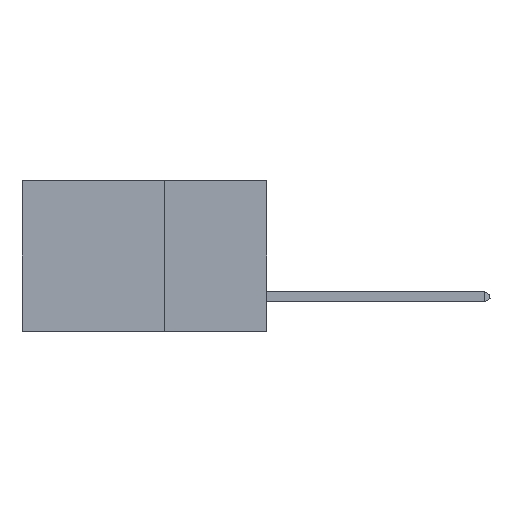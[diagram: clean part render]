
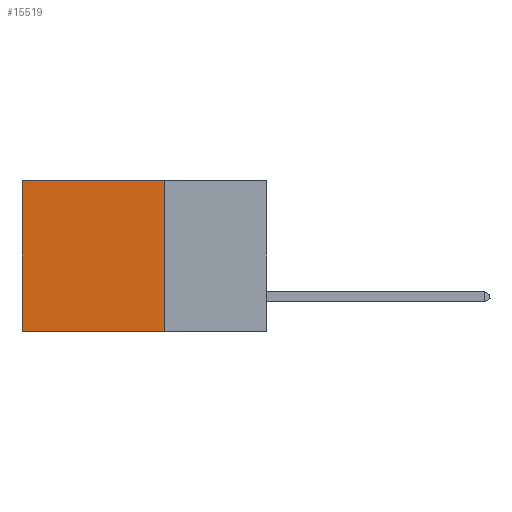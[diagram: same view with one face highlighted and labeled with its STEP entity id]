
A CAD part, left-side view. The second image highlights one B-rep face of the part: STEP entity #15519.
In plain terms, the highlighted planar face has unit normal (-1, 0, 0).
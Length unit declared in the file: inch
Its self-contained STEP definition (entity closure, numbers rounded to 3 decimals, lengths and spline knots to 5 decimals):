
#2589 = CARTESIAN_POINT ( 'NONE',  ( 0.2875, 0.25, 0. ) ) ;
#2641 = EDGE_CURVE ( 'NONE', #3528, #26989, #29992, .T. ) ;
#2643 = ORIENTED_EDGE ( 'NONE', *, *, #5439, .F. ) ;
#2852 = EDGE_LOOP ( 'NONE', ( #26876, #43610, #2643, #17409 ) ) ;
#3528 = VERTEX_POINT ( 'NONE', #34507 ) ;
#4433 = DIRECTION ( 'NONE',  ( 0., 0., -1. ) ) ;
#5439 = EDGE_CURVE ( 'NONE', #40015, #28971, #33391, .T. ) ;
#5545 = PLANE ( 'NONE',  #27857 ) ;
#6018 = LINE ( 'NONE', #2589, #21138 ) ;
#8181 = CARTESIAN_POINT ( 'NONE',  ( 0.2875, 0.25, 0. ) ) ;
#11436 = DIRECTION ( 'NONE',  ( 0., 0., -1. ) ) ;
#14682 = LINE ( 'NONE', #43186, #42162 ) ;
#15519 = ADVANCED_FACE ( 'NONE', ( #30611 ), #5545, .F. ) ;
#17409 = ORIENTED_EDGE ( 'NONE', *, *, #41048, .T. ) ;
#18837 = VECTOR ( 'NONE', #20607, 39.37008 ) ;
#20309 = CARTESIAN_POINT ( 'NONE',  ( 0.2875, 0.6, 0. ) ) ;
#20607 = DIRECTION ( 'NONE',  ( 0., 0., -1. ) ) ;
#21138 = VECTOR ( 'NONE', #42361, 39.37008 ) ;
#23609 = CARTESIAN_POINT ( 'NONE',  ( 0.2875, 0.25, 0. ) ) ;
#26876 = ORIENTED_EDGE ( 'NONE', *, *, #2641, .T. ) ;
#26989 = VERTEX_POINT ( 'NONE', #33875 ) ;
#27857 = AXIS2_PLACEMENT_3D ( 'NONE', #8181, #36940, #4433 ) ;
#28971 = VERTEX_POINT ( 'NONE', #38961 ) ;
#29795 = EDGE_CURVE ( 'NONE', #28971, #26989, #14682, .T. ) ;
#29992 = LINE ( 'NONE', #20309, #32766 ) ;
#30611 = FACE_OUTER_BOUND ( 'NONE', #2852, .T. ) ;
#32766 = VECTOR ( 'NONE', #11436, 39.37008 ) ;
#33391 = LINE ( 'NONE', #23609, #18837 ) ;
#33875 = CARTESIAN_POINT ( 'NONE',  ( 0.2875, 0.6, -0.37 ) ) ;
#34507 = CARTESIAN_POINT ( 'NONE',  ( 0.2875, 0.6, 0. ) ) ;
#35625 = DIRECTION ( 'NONE',  ( 0., 1., 0. ) ) ;
#36104 = CARTESIAN_POINT ( 'NONE',  ( 0.2875, 0.25, 0. ) ) ;
#36940 = DIRECTION ( 'NONE',  ( 1., 0., 0. ) ) ;
#38961 = CARTESIAN_POINT ( 'NONE',  ( 0.2875, 0.25, -0.37 ) ) ;
#40015 = VERTEX_POINT ( 'NONE', #36104 ) ;
#41048 = EDGE_CURVE ( 'NONE', #40015, #3528, #6018, .T. ) ;
#42162 = VECTOR ( 'NONE', #35625, 39.37008 ) ;
#42361 = DIRECTION ( 'NONE',  ( 0., 1., 0. ) ) ;
#43186 = CARTESIAN_POINT ( 'NONE',  ( 0.2875, 0.25, -0.37 ) ) ;
#43610 = ORIENTED_EDGE ( 'NONE', *, *, #29795, .F. ) ;
